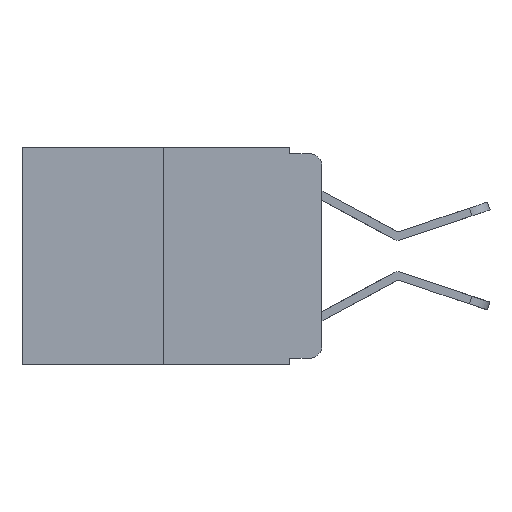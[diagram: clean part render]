
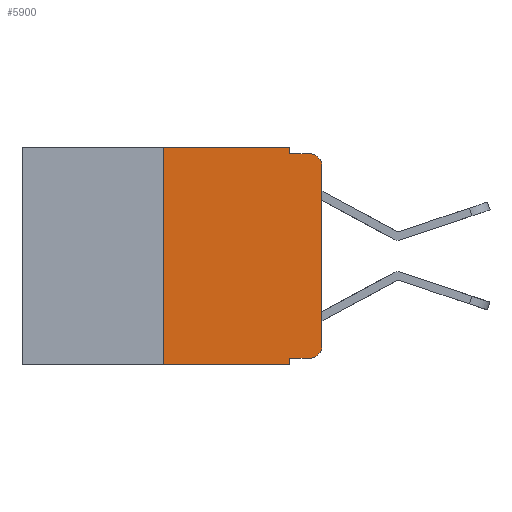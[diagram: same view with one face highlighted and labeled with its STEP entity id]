
A CAD part, left-side view. The second image highlights one B-rep face of the part: STEP entity #5900.
In plain terms, the highlighted planar face has unit normal (-1, 0, 0).
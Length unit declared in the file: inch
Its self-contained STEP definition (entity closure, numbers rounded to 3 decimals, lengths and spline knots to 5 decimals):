
#546 = CARTESIAN_POINT ( 'NONE',  ( 0., 0.25, -0.343 ) ) ;
#958 = EDGE_LOOP ( 'NONE', ( #3326, #6202, #6857, #4396, #5409, #8127, #13437, #2776, #6048, #11701 ) ) ;
#1028 = AXIS2_PLACEMENT_3D ( 'NONE', #10448, #4338, #11444 ) ;
#1031 = DIRECTION ( 'NONE',  ( 0., 0., -1. ) ) ;
#1038 = EDGE_CURVE ( 'NONE', #10566, #12806, #6981, .T. ) ;
#1067 = FACE_OUTER_BOUND ( 'NONE', #958, .T. ) ;
#1082 = LINE ( 'NONE', #6970, #6916 ) ;
#1128 = CARTESIAN_POINT ( 'NONE',  ( 0., 0.02, -0.03 ) ) ;
#1169 = CARTESIAN_POINT ( 'NONE',  ( 0., 0., -0.313 ) ) ;
#1837 = CARTESIAN_POINT ( 'NONE',  ( 0., 0.25, 0. ) ) ;
#2044 = CARTESIAN_POINT ( 'NONE',  ( 0., 0.051, -0.01 ) ) ;
#2288 = DIRECTION ( 'NONE',  ( 0., 0., -1. ) ) ;
#2554 = EDGE_CURVE ( 'NONE', #10566, #12941, #2892, .T. ) ;
#2654 = DIRECTION ( 'NONE',  ( 0., 0., -1. ) ) ;
#2776 = ORIENTED_EDGE ( 'NONE', *, *, #11419, .F. ) ;
#2892 = LINE ( 'NONE', #10606, #13533 ) ;
#3106 = AXIS2_PLACEMENT_3D ( 'NONE', #13529, #7541, #1031 ) ;
#3326 = ORIENTED_EDGE ( 'NONE', *, *, #10496, .T. ) ;
#4032 = CARTESIAN_POINT ( 'NONE',  ( 0., 0.051, 0. ) ) ;
#4338 = DIRECTION ( 'NONE',  ( -1., 0., 0. ) ) ;
#4389 = CARTESIAN_POINT ( 'NONE',  ( 0., 0.051, 0. ) ) ;
#4396 = ORIENTED_EDGE ( 'NONE', *, *, #9363, .F. ) ;
#4460 = LINE ( 'NONE', #10941, #6599 ) ;
#4553 = EDGE_CURVE ( 'NONE', #5850, #10080, #7224, .T. ) ;
#4746 = VERTEX_POINT ( 'NONE', #1169 ) ;
#5015 = DIRECTION ( 'NONE',  ( 0., 0., 1. ) ) ;
#5080 = VERTEX_POINT ( 'NONE', #9273 ) ;
#5148 = VERTEX_POINT ( 'NONE', #6358 ) ;
#5165 = VECTOR ( 'NONE', #5015, 39.37008 ) ;
#5409 = ORIENTED_EDGE ( 'NONE', *, *, #11418, .F. ) ;
#5850 = VERTEX_POINT ( 'NONE', #2044 ) ;
#5900 = ADVANCED_FACE ( 'NONE', ( #1067 ), #12535, .F. ) ;
#6021 = DIRECTION ( 'NONE',  ( 0., 0., 1. ) ) ;
#6048 = ORIENTED_EDGE ( 'NONE', *, *, #12591, .T. ) ;
#6064 = DIRECTION ( 'NONE',  ( 0., -1., 0. ) ) ;
#6148 = VERTEX_POINT ( 'NONE', #12898 ) ;
#6149 = VECTOR ( 'NONE', #13154, 39.37008 ) ;
#6202 = ORIENTED_EDGE ( 'NONE', *, *, #12283, .T. ) ;
#6358 = CARTESIAN_POINT ( 'NONE',  ( 0., 0.02, -0.333 ) ) ;
#6463 = EDGE_CURVE ( 'NONE', #5148, #4746, #12680, .T. ) ;
#6556 = CIRCLE ( 'NONE', #12893, 0.02 ) ;
#6599 = VECTOR ( 'NONE', #2654, 39.37008 ) ;
#6857 = ORIENTED_EDGE ( 'NONE', *, *, #4553, .F. ) ;
#6913 = VECTOR ( 'NONE', #10313, 39.37008 ) ;
#6916 = VECTOR ( 'NONE', #7996, 39.37008 ) ;
#6970 = CARTESIAN_POINT ( 'NONE',  ( 0., 0.473, 0. ) ) ;
#6981 = LINE ( 'NONE', #1837, #12304 ) ;
#7224 = LINE ( 'NONE', #12103, #6913 ) ;
#7541 = DIRECTION ( 'NONE',  ( 1., 0., 0. ) ) ;
#7666 = CARTESIAN_POINT ( 'NONE',  ( 0., 0.051, -0.343 ) ) ;
#7996 = DIRECTION ( 'NONE',  ( 0., -1., 0. ) ) ;
#8127 = ORIENTED_EDGE ( 'NONE', *, *, #1038, .F. ) ;
#8650 = LINE ( 'NONE', #9123, #13312 ) ;
#8668 = DIRECTION ( 'NONE',  ( -1., 0., 0. ) ) ;
#8800 = DIRECTION ( 'NONE',  ( 0., -1., 0. ) ) ;
#9123 = CARTESIAN_POINT ( 'NONE',  ( 0., 0.051, -0.333 ) ) ;
#9273 = CARTESIAN_POINT ( 'NONE',  ( 0., 0.051, -0.333 ) ) ;
#9363 = EDGE_CURVE ( 'NONE', #9578, #5850, #13528, .T. ) ;
#9578 = VERTEX_POINT ( 'NONE', #4389 ) ;
#10080 = VERTEX_POINT ( 'NONE', #10428 ) ;
#10313 = DIRECTION ( 'NONE',  ( 0., -1., 0. ) ) ;
#10428 = CARTESIAN_POINT ( 'NONE',  ( 0., 0.02, -0.01 ) ) ;
#10448 = CARTESIAN_POINT ( 'NONE',  ( 0., 0.02, -0.313 ) ) ;
#10496 = EDGE_CURVE ( 'NONE', #4746, #6148, #10541, .T. ) ;
#10541 = LINE ( 'NONE', #11070, #5165 ) ;
#10566 = VERTEX_POINT ( 'NONE', #546 ) ;
#10606 = CARTESIAN_POINT ( 'NONE',  ( 0., 0.473, -0.343 ) ) ;
#10941 = CARTESIAN_POINT ( 'NONE',  ( 0., 0.051, 0. ) ) ;
#11070 = CARTESIAN_POINT ( 'NONE',  ( 0., 0., 0. ) ) ;
#11415 = CARTESIAN_POINT ( 'NONE',  ( 0., 0.25, 0. ) ) ;
#11418 = EDGE_CURVE ( 'NONE', #12806, #9578, #1082, .T. ) ;
#11419 = EDGE_CURVE ( 'NONE', #5080, #12941, #4460, .T. ) ;
#11444 = DIRECTION ( 'NONE',  ( 0., 0., -1. ) ) ;
#11701 = ORIENTED_EDGE ( 'NONE', *, *, #6463, .T. ) ;
#12103 = CARTESIAN_POINT ( 'NONE',  ( 0., 0.051, -0.01 ) ) ;
#12283 = EDGE_CURVE ( 'NONE', #6148, #10080, #6556, .T. ) ;
#12304 = VECTOR ( 'NONE', #6021, 39.37008 ) ;
#12535 = PLANE ( 'NONE',  #3106 ) ;
#12591 = EDGE_CURVE ( 'NONE', #5080, #5148, #8650, .T. ) ;
#12680 = CIRCLE ( 'NONE', #1028, 0.02 ) ;
#12806 = VERTEX_POINT ( 'NONE', #11415 ) ;
#12893 = AXIS2_PLACEMENT_3D ( 'NONE', #1128, #8668, #2288 ) ;
#12898 = CARTESIAN_POINT ( 'NONE',  ( 0., 0., -0.03 ) ) ;
#12941 = VERTEX_POINT ( 'NONE', #7666 ) ;
#13154 = DIRECTION ( 'NONE',  ( 0., 0., -1. ) ) ;
#13312 = VECTOR ( 'NONE', #6064, 39.37008 ) ;
#13437 = ORIENTED_EDGE ( 'NONE', *, *, #2554, .T. ) ;
#13528 = LINE ( 'NONE', #4032, #6149 ) ;
#13529 = CARTESIAN_POINT ( 'NONE',  ( 0., 0.473, 0. ) ) ;
#13533 = VECTOR ( 'NONE', #8800, 39.37008 ) ;
